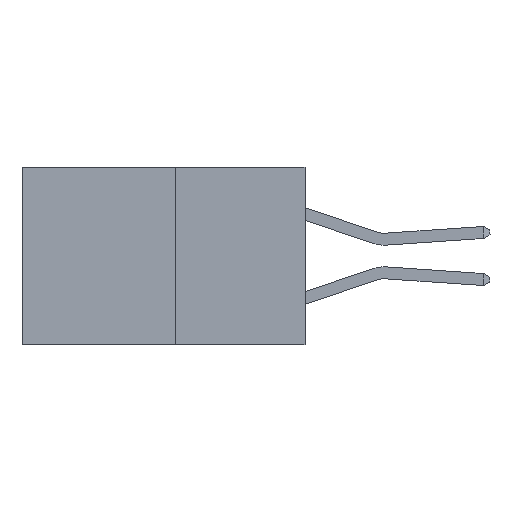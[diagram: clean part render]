
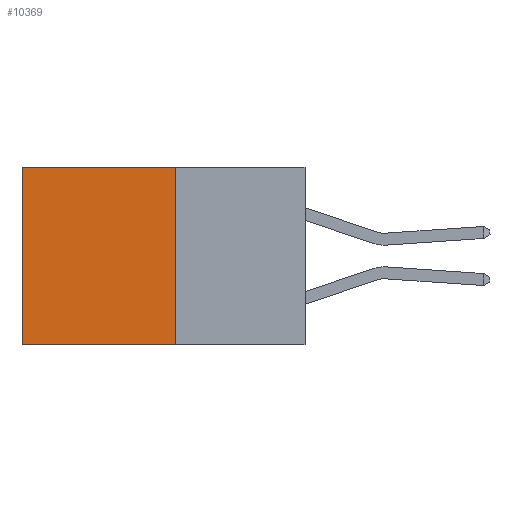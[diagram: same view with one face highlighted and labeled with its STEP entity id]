
A CAD part, left-side view. The second image highlights one B-rep face of the part: STEP entity #10369.
In plain terms, the highlighted planar face has unit normal (-1, 0, 0).
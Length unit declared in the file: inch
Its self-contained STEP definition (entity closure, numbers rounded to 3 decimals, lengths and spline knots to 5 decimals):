
#34 = LINE ( 'NONE', #10052, #16307 ) ;
#339 = CARTESIAN_POINT ( 'NONE',  ( 0.277, 0.59, -0.37 ) ) ;
#377 = CARTESIAN_POINT ( 'NONE',  ( 0.277, 0.27, -0.37 ) ) ;
#602 = VERTEX_POINT ( 'NONE', #15989 ) ;
#1000 = ORIENTED_EDGE ( 'NONE', *, *, #17045, .T. ) ;
#1090 = EDGE_LOOP ( 'NONE', ( #1000, #13111, #3446, #15844 ) ) ;
#1272 = CARTESIAN_POINT ( 'NONE',  ( 0.277, 0.27, -0.37 ) ) ;
#1839 = CARTESIAN_POINT ( 'NONE',  ( 0.277, 0.27, -0.37 ) ) ;
#1842 = FACE_OUTER_BOUND ( 'NONE', #1090, .T. ) ;
#1951 = LINE ( 'NONE', #339, #10105 ) ;
#3446 = ORIENTED_EDGE ( 'NONE', *, *, #9507, .F. ) ;
#3778 = DIRECTION ( 'NONE',  ( 0., 0., -1. ) ) ;
#5146 = DIRECTION ( 'NONE',  ( 0., 0., -1. ) ) ;
#5515 = DIRECTION ( 'NONE',  ( 0., 0., -1. ) ) ;
#6037 = LINE ( 'NONE', #1272, #6553 ) ;
#6553 = VECTOR ( 'NONE', #5515, 39.37008 ) ;
#7031 = VERTEX_POINT ( 'NONE', #16999 ) ;
#7530 = EDGE_CURVE ( 'NONE', #14703, #7031, #34, .T. ) ;
#9507 = EDGE_CURVE ( 'NONE', #602, #14703, #6037, .T. ) ;
#9851 = DIRECTION ( 'NONE',  ( 0., 1., 0. ) ) ;
#10052 = CARTESIAN_POINT ( 'NONE',  ( 0.277, 0.27, -0.37 ) ) ;
#10105 = VECTOR ( 'NONE', #3778, 39.37008 ) ;
#10369 = ADVANCED_FACE ( 'NONE', ( #1842 ), #11606, .F. ) ;
#10903 = CARTESIAN_POINT ( 'NONE',  ( 0.277, 0.59, 0. ) ) ;
#11606 = PLANE ( 'NONE',  #17421 ) ;
#11617 = LINE ( 'NONE', #14847, #14379 ) ;
#12753 = VERTEX_POINT ( 'NONE', #10903 ) ;
#13111 = ORIENTED_EDGE ( 'NONE', *, *, #7530, .F. ) ;
#14379 = VECTOR ( 'NONE', #19514, 39.37008 ) ;
#14703 = VERTEX_POINT ( 'NONE', #377 ) ;
#14827 = DIRECTION ( 'NONE',  ( 1., 0., 0. ) ) ;
#14847 = CARTESIAN_POINT ( 'NONE',  ( 0.277, 0.27, 0. ) ) ;
#15844 = ORIENTED_EDGE ( 'NONE', *, *, #18168, .T. ) ;
#15989 = CARTESIAN_POINT ( 'NONE',  ( 0.277, 0.27, 0. ) ) ;
#16307 = VECTOR ( 'NONE', #9851, 39.37008 ) ;
#16999 = CARTESIAN_POINT ( 'NONE',  ( 0.277, 0.59, -0.37 ) ) ;
#17045 = EDGE_CURVE ( 'NONE', #12753, #7031, #1951, .T. ) ;
#17421 = AXIS2_PLACEMENT_3D ( 'NONE', #1839, #14827, #5146 ) ;
#18168 = EDGE_CURVE ( 'NONE', #602, #12753, #11617, .T. ) ;
#19514 = DIRECTION ( 'NONE',  ( 0., 1., 0. ) ) ;
